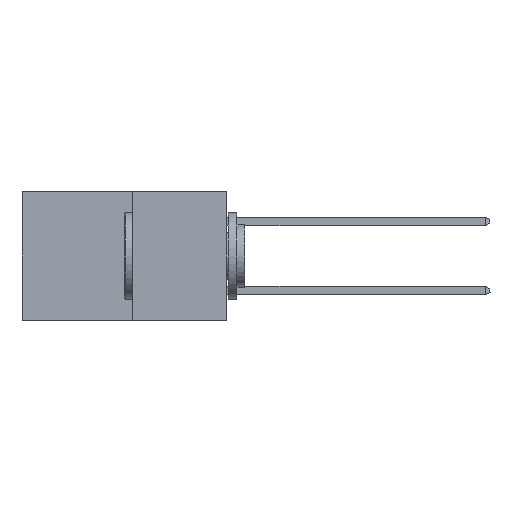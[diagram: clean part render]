
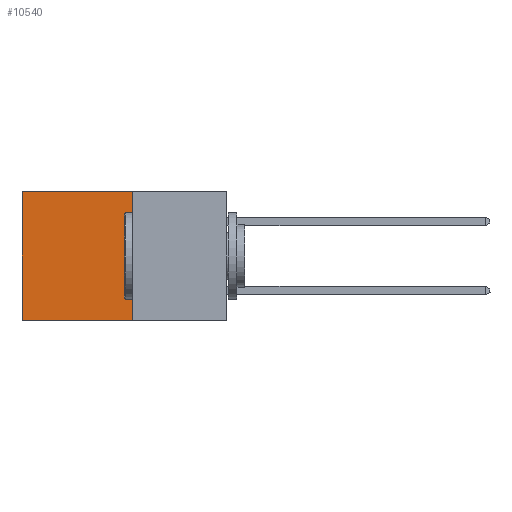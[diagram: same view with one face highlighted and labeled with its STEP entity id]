
A CAD part, left-side view. The second image highlights one B-rep face of the part: STEP entity #10540.
In plain terms, the highlighted planar face has unit normal (-1, 0, 0).
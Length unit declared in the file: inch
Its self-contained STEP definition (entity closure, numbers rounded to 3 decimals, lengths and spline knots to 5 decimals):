
#3 = CARTESIAN_POINT ( 'NONE',  ( 0.277, 0.27, 0. ) ) ;
#570 = EDGE_LOOP ( 'NONE', ( #10159, #10408, #8703, #2663 ) ) ;
#1142 = LINE ( 'NONE', #3, #7886 ) ;
#2212 = VERTEX_POINT ( 'NONE', #2274 ) ;
#2274 = CARTESIAN_POINT ( 'NONE',  ( 0.277, 0.59, 0. ) ) ;
#2528 = CARTESIAN_POINT ( 'NONE',  ( 0.277, 0.27, -0.37 ) ) ;
#2604 = FACE_OUTER_BOUND ( 'NONE', #570, .T. ) ;
#2663 = ORIENTED_EDGE ( 'NONE', *, *, #3695, .T. ) ;
#3002 = EDGE_CURVE ( 'NONE', #4117, #9770, #3369, .T. ) ;
#3109 = VECTOR ( 'NONE', #8095, 39.37008 ) ;
#3369 = LINE ( 'NONE', #6457, #7266 ) ;
#3381 = DIRECTION ( 'NONE',  ( 0., 0., -1. ) ) ;
#3695 = EDGE_CURVE ( 'NONE', #4504, #2212, #1142, .T. ) ;
#3783 = CARTESIAN_POINT ( 'NONE',  ( 0.277, 0.27, -0.37 ) ) ;
#4117 = VERTEX_POINT ( 'NONE', #3783 ) ;
#4280 = LINE ( 'NONE', #9923, #8376 ) ;
#4504 = VERTEX_POINT ( 'NONE', #9413 ) ;
#4689 = EDGE_CURVE ( 'NONE', #2212, #9770, #9616, .T. ) ;
#5412 = AXIS2_PLACEMENT_3D ( 'NONE', #2528, #8311, #3381 ) ;
#6289 = EDGE_CURVE ( 'NONE', #4504, #4117, #4280, .T. ) ;
#6457 = CARTESIAN_POINT ( 'NONE',  ( 0.277, 0.27, -0.37 ) ) ;
#6702 = PLANE ( 'NONE',  #5412 ) ;
#6742 = DIRECTION ( 'NONE',  ( 0., 1., 0. ) ) ;
#7266 = VECTOR ( 'NONE', #6742, 39.37008 ) ;
#7886 = VECTOR ( 'NONE', #8027, 39.37008 ) ;
#8027 = DIRECTION ( 'NONE',  ( 0., 1., 0. ) ) ;
#8073 = CARTESIAN_POINT ( 'NONE',  ( 0.277, 0.59, -0.37 ) ) ;
#8095 = DIRECTION ( 'NONE',  ( 0., 0., -1. ) ) ;
#8311 = DIRECTION ( 'NONE',  ( 1., 0., 0. ) ) ;
#8376 = VECTOR ( 'NONE', #9836, 39.37008 ) ;
#8703 = ORIENTED_EDGE ( 'NONE', *, *, #6289, .F. ) ;
#9413 = CARTESIAN_POINT ( 'NONE',  ( 0.277, 0.27, 0. ) ) ;
#9616 = LINE ( 'NONE', #8073, #3109 ) ;
#9770 = VERTEX_POINT ( 'NONE', #10608 ) ;
#9836 = DIRECTION ( 'NONE',  ( 0., 0., -1. ) ) ;
#9923 = CARTESIAN_POINT ( 'NONE',  ( 0.277, 0.27, -0.37 ) ) ;
#10159 = ORIENTED_EDGE ( 'NONE', *, *, #4689, .T. ) ;
#10408 = ORIENTED_EDGE ( 'NONE', *, *, #3002, .F. ) ;
#10540 = ADVANCED_FACE ( 'NONE', ( #2604 ), #6702, .F. ) ;
#10608 = CARTESIAN_POINT ( 'NONE',  ( 0.277, 0.59, -0.37 ) ) ;
